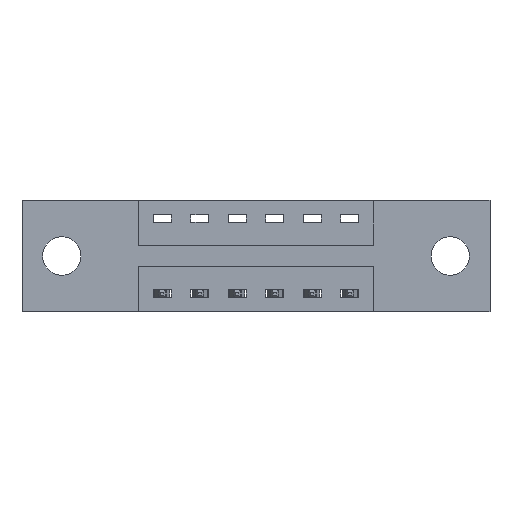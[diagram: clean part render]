
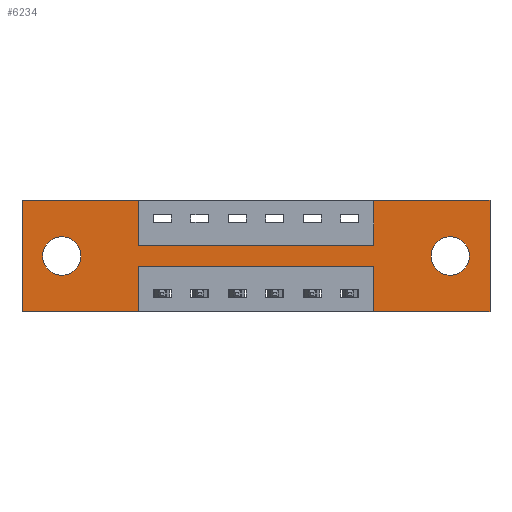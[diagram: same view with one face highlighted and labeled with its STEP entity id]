
A CAD part, front view. The second image highlights one B-rep face of the part: STEP entity #6234.
In plain terms, the highlighted planar face has unit normal (0, -1, 0).
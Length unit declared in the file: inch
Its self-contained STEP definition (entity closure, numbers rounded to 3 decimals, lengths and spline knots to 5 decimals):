
#85 = EDGE_CURVE ( 'NONE', #3641, #1362, #1662, .T. ) ;
#233 = EDGE_CURVE ( 'NONE', #7707, #2812, #601, .T. ) ;
#316 = CIRCLE ( 'NONE', #5445, 0.064 ) ;
#328 = VERTEX_POINT ( 'NONE', #4592 ) ;
#358 = VECTOR ( 'NONE', #6749, 39.37008 ) ;
#359 = EDGE_LOOP ( 'NONE', ( #5367, #7112 ) ) ;
#366 = VERTEX_POINT ( 'NONE', #5330 ) ;
#405 = AXIS2_PLACEMENT_3D ( 'NONE', #5272, #7691, #6513 ) ;
#444 = ORIENTED_EDGE ( 'NONE', *, *, #7767, .F. ) ;
#593 = DIRECTION ( 'NONE',  ( 0., 0., -1. ) ) ;
#601 = CIRCLE ( 'NONE', #405, 0.064 ) ;
#606 = EDGE_LOOP ( 'NONE', ( #5167, #6931 ) ) ;
#652 = ORIENTED_EDGE ( 'NONE', *, *, #1873, .F. ) ;
#792 = AXIS2_PLACEMENT_3D ( 'NONE', #2268, #2929, #7566 ) ;
#829 = FACE_BOUND ( 'NONE', #359, .T. ) ;
#943 = VECTOR ( 'NONE', #7320, 39.37008 ) ;
#954 = LINE ( 'NONE', #1562, #4338 ) ;
#1156 = LINE ( 'NONE', #4697, #943 ) ;
#1229 = CARTESIAN_POINT ( 'NONE',  ( 1.56, 0., -0.37 ) ) ;
#1258 = CARTESIAN_POINT ( 'NONE',  ( 1.1725, 0., -0.15 ) ) ;
#1362 = VERTEX_POINT ( 'NONE', #5517 ) ;
#1376 = CARTESIAN_POINT ( 'NONE',  ( 1.1725, 0., 0. ) ) ;
#1392 = CARTESIAN_POINT ( 'NONE',  ( 0.3875, 0., -0.22 ) ) ;
#1513 = CARTESIAN_POINT ( 'NONE',  ( 1.4275, 0., -0.249 ) ) ;
#1544 = VECTOR ( 'NONE', #593, 39.37008 ) ;
#1562 = CARTESIAN_POINT ( 'NONE',  ( 0., 0., -0.37 ) ) ;
#1662 = LINE ( 'NONE', #8069, #5424 ) ;
#1696 = VERTEX_POINT ( 'NONE', #1392 ) ;
#1815 = LINE ( 'NONE', #2189, #8250 ) ;
#1873 = EDGE_CURVE ( 'NONE', #4443, #5825, #3565, .T. ) ;
#1906 = VECTOR ( 'NONE', #3976, 39.37008 ) ;
#2021 = ORIENTED_EDGE ( 'NONE', *, *, #6970, .F. ) ;
#2087 = VECTOR ( 'NONE', #6916, 39.37008 ) ;
#2099 = VECTOR ( 'NONE', #7398, 39.37008 ) ;
#2189 = CARTESIAN_POINT ( 'NONE',  ( 0., 0., 0. ) ) ;
#2237 = ORIENTED_EDGE ( 'NONE', *, *, #5956, .F. ) ;
#2268 = CARTESIAN_POINT ( 'NONE',  ( 0., 0., -0.37 ) ) ;
#2364 = VERTEX_POINT ( 'NONE', #3260 ) ;
#2509 = CARTESIAN_POINT ( 'NONE',  ( 0., 0., 0. ) ) ;
#2584 = EDGE_CURVE ( 'NONE', #2364, #328, #6343, .T. ) ;
#2693 = DIRECTION ( 'NONE',  ( 0., 0., 1. ) ) ;
#2705 = CARTESIAN_POINT ( 'NONE',  ( 1.4275, 0., -0.121 ) ) ;
#2734 = CARTESIAN_POINT ( 'NONE',  ( 0.3875, 0., -0.37 ) ) ;
#2754 = CARTESIAN_POINT ( 'NONE',  ( 0., 0., 0. ) ) ;
#2761 = CARTESIAN_POINT ( 'NONE',  ( 0., 0., -0.37 ) ) ;
#2787 = CARTESIAN_POINT ( 'NONE',  ( 1.1725, 0., -0.37 ) ) ;
#2812 = VERTEX_POINT ( 'NONE', #1513 ) ;
#2815 = DIRECTION ( 'NONE',  ( 0., 0., 1. ) ) ;
#2874 = VECTOR ( 'NONE', #4838, 39.37008 ) ;
#2929 = DIRECTION ( 'NONE',  ( 0., -1., 0. ) ) ;
#2991 = CARTESIAN_POINT ( 'NONE',  ( 0.1325, 0., -0.185 ) ) ;
#3021 = CARTESIAN_POINT ( 'NONE',  ( 1.1725, 0., 0. ) ) ;
#3107 = LINE ( 'NONE', #3021, #4701 ) ;
#3258 = EDGE_CURVE ( 'NONE', #5880, #6011, #3107, .T. ) ;
#3260 = CARTESIAN_POINT ( 'NONE',  ( 0.1325, 0., -0.249 ) ) ;
#3475 = DIRECTION ( 'NONE',  ( 0., 1., 0. ) ) ;
#3502 = LINE ( 'NONE', #7887, #1906 ) ;
#3555 = VERTEX_POINT ( 'NONE', #2734 ) ;
#3565 = LINE ( 'NONE', #6734, #1544 ) ;
#3641 = VERTEX_POINT ( 'NONE', #2787 ) ;
#3841 = ORIENTED_EDGE ( 'NONE', *, *, #7189, .F. ) ;
#3896 = AXIS2_PLACEMENT_3D ( 'NONE', #2991, #5622, #2815 ) ;
#3976 = DIRECTION ( 'NONE',  ( 1., 0., 0. ) ) ;
#4044 = ORIENTED_EDGE ( 'NONE', *, *, #6067, .F. ) ;
#4068 = EDGE_CURVE ( 'NONE', #2812, #7707, #6531, .T. ) ;
#4165 = LINE ( 'NONE', #2761, #358 ) ;
#4255 = ORIENTED_EDGE ( 'NONE', *, *, #8469, .F. ) ;
#4338 = VECTOR ( 'NONE', #8206, 39.37008 ) ;
#4430 = FACE_OUTER_BOUND ( 'NONE', #4933, .T. ) ;
#4439 = VECTOR ( 'NONE', #6501, 39.37008 ) ;
#4443 = VERTEX_POINT ( 'NONE', #8451 ) ;
#4584 = DIRECTION ( 'NONE',  ( 0., 0., -1. ) ) ;
#4592 = CARTESIAN_POINT ( 'NONE',  ( 0.1325, 0., -0.121 ) ) ;
#4605 = CARTESIAN_POINT ( 'NONE',  ( 0.3875, 0., -0.15 ) ) ;
#4690 = LINE ( 'NONE', #6781, #2874 ) ;
#4697 = CARTESIAN_POINT ( 'NONE',  ( 1.56, 0., 0. ) ) ;
#4701 = VECTOR ( 'NONE', #2693, 39.37008 ) ;
#4838 = DIRECTION ( 'NONE',  ( -1., 0., 0. ) ) ;
#4843 = FACE_BOUND ( 'NONE', #606, .T. ) ;
#4933 = EDGE_LOOP ( 'NONE', ( #2021, #3841, #7331, #444, #2237, #4044, #5783, #7525, #652, #4255, #6008, #7721 ) ) ;
#5145 = EDGE_CURVE ( 'NONE', #5825, #5880, #3502, .T. ) ;
#5167 = ORIENTED_EDGE ( 'NONE', *, *, #233, .T. ) ;
#5272 = CARTESIAN_POINT ( 'NONE',  ( 1.4275, 0., -0.185 ) ) ;
#5330 = CARTESIAN_POINT ( 'NONE',  ( 0., 0., 0. ) ) ;
#5367 = ORIENTED_EDGE ( 'NONE', *, *, #6088, .T. ) ;
#5424 = VECTOR ( 'NONE', #8236, 39.37008 ) ;
#5445 = AXIS2_PLACEMENT_3D ( 'NONE', #7429, #3475, #8081 ) ;
#5489 = EDGE_CURVE ( 'NONE', #3555, #8265, #954, .T. ) ;
#5517 = CARTESIAN_POINT ( 'NONE',  ( 1.1725, 0., -0.22 ) ) ;
#5622 = DIRECTION ( 'NONE',  ( 0., 1., 0. ) ) ;
#5654 = LINE ( 'NONE', #2754, #2099 ) ;
#5743 = EDGE_CURVE ( 'NONE', #8265, #366, #7702, .T. ) ;
#5783 = ORIENTED_EDGE ( 'NONE', *, *, #3258, .F. ) ;
#5825 = VERTEX_POINT ( 'NONE', #4605 ) ;
#5880 = VERTEX_POINT ( 'NONE', #1258 ) ;
#5940 = CARTESIAN_POINT ( 'NONE',  ( 0., 0., -0.37 ) ) ;
#5956 = EDGE_CURVE ( 'NONE', #6456, #8238, #1156, .T. ) ;
#6008 = ORIENTED_EDGE ( 'NONE', *, *, #5743, .F. ) ;
#6011 = VERTEX_POINT ( 'NONE', #1376 ) ;
#6012 = AXIS2_PLACEMENT_3D ( 'NONE', #8319, #7830, #4584 ) ;
#6067 = EDGE_CURVE ( 'NONE', #6011, #6456, #5654, .T. ) ;
#6088 = EDGE_CURVE ( 'NONE', #328, #2364, #316, .T. ) ;
#6196 = DIRECTION ( 'NONE',  ( 1., 0., 0. ) ) ;
#6234 = ADVANCED_FACE ( 'NONE', ( #4843, #829, #4430 ), #6256, .T. ) ;
#6256 = PLANE ( 'NONE',  #792 ) ;
#6343 = CIRCLE ( 'NONE', #3896, 0.064 ) ;
#6456 = VERTEX_POINT ( 'NONE', #8450 ) ;
#6501 = DIRECTION ( 'NONE',  ( 0., 0., 1. ) ) ;
#6513 = DIRECTION ( 'NONE',  ( 0., 0., -1. ) ) ;
#6531 = CIRCLE ( 'NONE', #6012, 0.064 ) ;
#6734 = CARTESIAN_POINT ( 'NONE',  ( 0.3875, 0., 0. ) ) ;
#6749 = DIRECTION ( 'NONE',  ( -1., 0., 0. ) ) ;
#6781 = CARTESIAN_POINT ( 'NONE',  ( 0.3875, 0., -0.22 ) ) ;
#6916 = DIRECTION ( 'NONE',  ( 0., 0., -1. ) ) ;
#6931 = ORIENTED_EDGE ( 'NONE', *, *, #4068, .T. ) ;
#6970 = EDGE_CURVE ( 'NONE', #1696, #3555, #7786, .T. ) ;
#7112 = ORIENTED_EDGE ( 'NONE', *, *, #2584, .T. ) ;
#7189 = EDGE_CURVE ( 'NONE', #1362, #1696, #4690, .T. ) ;
#7320 = DIRECTION ( 'NONE',  ( 0., 0., -1. ) ) ;
#7331 = ORIENTED_EDGE ( 'NONE', *, *, #85, .F. ) ;
#7398 = DIRECTION ( 'NONE',  ( 1., 0., 0. ) ) ;
#7429 = CARTESIAN_POINT ( 'NONE',  ( 0.1325, 0., -0.185 ) ) ;
#7525 = ORIENTED_EDGE ( 'NONE', *, *, #5145, .F. ) ;
#7566 = DIRECTION ( 'NONE',  ( 0., 0., -1. ) ) ;
#7691 = DIRECTION ( 'NONE',  ( 0., 1., 0. ) ) ;
#7702 = LINE ( 'NONE', #2509, #4439 ) ;
#7707 = VERTEX_POINT ( 'NONE', #2705 ) ;
#7721 = ORIENTED_EDGE ( 'NONE', *, *, #5489, .F. ) ;
#7767 = EDGE_CURVE ( 'NONE', #8238, #3641, #4165, .T. ) ;
#7786 = LINE ( 'NONE', #8185, #2087 ) ;
#7830 = DIRECTION ( 'NONE',  ( 0., 1., 0. ) ) ;
#7887 = CARTESIAN_POINT ( 'NONE',  ( 0.3875, 0., -0.15 ) ) ;
#8069 = CARTESIAN_POINT ( 'NONE',  ( 1.1725, 0., -0.37 ) ) ;
#8081 = DIRECTION ( 'NONE',  ( 0., 0., 1. ) ) ;
#8185 = CARTESIAN_POINT ( 'NONE',  ( 0.3875, 0., -0.37 ) ) ;
#8206 = DIRECTION ( 'NONE',  ( -1., 0., 0. ) ) ;
#8236 = DIRECTION ( 'NONE',  ( 0., 0., 1. ) ) ;
#8238 = VERTEX_POINT ( 'NONE', #1229 ) ;
#8250 = VECTOR ( 'NONE', #6196, 39.37008 ) ;
#8265 = VERTEX_POINT ( 'NONE', #5940 ) ;
#8319 = CARTESIAN_POINT ( 'NONE',  ( 1.4275, 0., -0.185 ) ) ;
#8450 = CARTESIAN_POINT ( 'NONE',  ( 1.56, 0., 0. ) ) ;
#8451 = CARTESIAN_POINT ( 'NONE',  ( 0.3875, 0., 0. ) ) ;
#8469 = EDGE_CURVE ( 'NONE', #366, #4443, #1815, .T. ) ;
